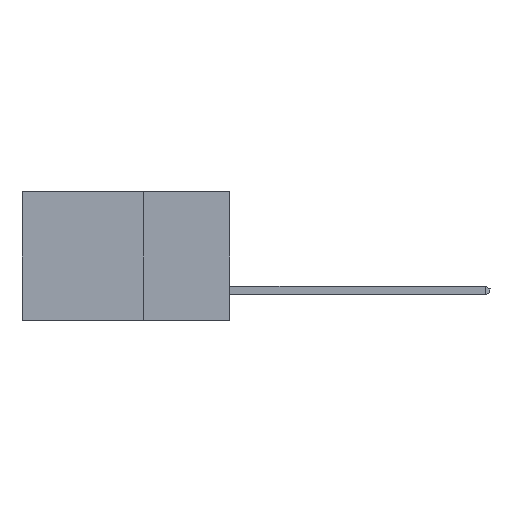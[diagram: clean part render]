
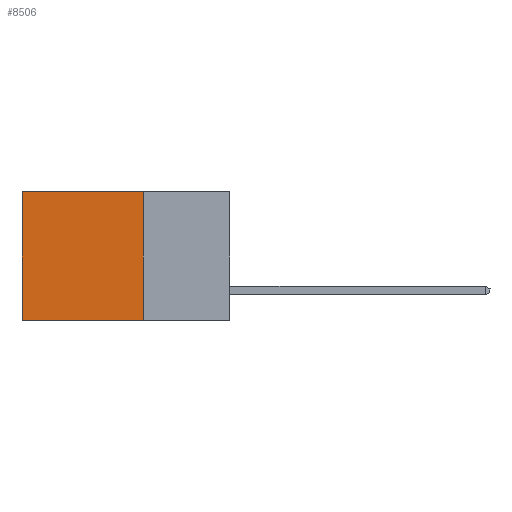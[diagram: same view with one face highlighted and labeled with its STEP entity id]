
A CAD part, left-side view. The second image highlights one B-rep face of the part: STEP entity #8506.
In plain terms, the highlighted planar face has unit normal (-1, 0, 0).
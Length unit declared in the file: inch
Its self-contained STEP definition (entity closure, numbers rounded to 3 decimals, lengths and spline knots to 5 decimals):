
#11 = EDGE_CURVE ( 'NONE', #2244, #3893, #8673, .T. ) ;
#474 = VECTOR ( 'NONE', #10063, 39.37008 ) ;
#539 = CARTESIAN_POINT ( 'NONE',  ( 0.2615, 0.25, -0.37 ) ) ;
#571 = LINE ( 'NONE', #3663, #9584 ) ;
#933 = LINE ( 'NONE', #4939, #4636 ) ;
#1692 = DIRECTION ( 'NONE',  ( 1., 0., 0. ) ) ;
#1859 = EDGE_CURVE ( 'NONE', #2244, #2149, #933, .T. ) ;
#2149 = VERTEX_POINT ( 'NONE', #4140 ) ;
#2244 = VERTEX_POINT ( 'NONE', #7410 ) ;
#2729 = ORIENTED_EDGE ( 'NONE', *, *, #6774, .T. ) ;
#2737 = CARTESIAN_POINT ( 'NONE',  ( 0.2615, 0.25, -0.37 ) ) ;
#2770 = DIRECTION ( 'NONE',  ( 0., 1., 0. ) ) ;
#2777 = CARTESIAN_POINT ( 'NONE',  ( 0.2615, 0.6, -0.37 ) ) ;
#3311 = EDGE_LOOP ( 'NONE', ( #2729, #11397, #3771, #11235 ) ) ;
#3663 = CARTESIAN_POINT ( 'NONE',  ( 0.2615, 0.6, -0.37 ) ) ;
#3712 = PLANE ( 'NONE',  #9403 ) ;
#3771 = ORIENTED_EDGE ( 'NONE', *, *, #11, .F. ) ;
#3893 = VERTEX_POINT ( 'NONE', #11339 ) ;
#4140 = CARTESIAN_POINT ( 'NONE',  ( 0.2615, 0.6, 0. ) ) ;
#4167 = EDGE_CURVE ( 'NONE', #3893, #5742, #5219, .T. ) ;
#4636 = VECTOR ( 'NONE', #2770, 39.37008 ) ;
#4939 = CARTESIAN_POINT ( 'NONE',  ( 0.2615, 0.25, 0. ) ) ;
#5219 = LINE ( 'NONE', #11192, #474 ) ;
#5742 = VERTEX_POINT ( 'NONE', #2777 ) ;
#6774 = EDGE_CURVE ( 'NONE', #2149, #5742, #571, .T. ) ;
#7410 = CARTESIAN_POINT ( 'NONE',  ( 0.2615, 0.25, 0. ) ) ;
#8486 = DIRECTION ( 'NONE',  ( 0., 0., -1. ) ) ;
#8506 = ADVANCED_FACE ( 'NONE', ( #12841 ), #3712, .F. ) ;
#8576 = DIRECTION ( 'NONE',  ( 0., 0., -1. ) ) ;
#8673 = LINE ( 'NONE', #539, #11702 ) ;
#9403 = AXIS2_PLACEMENT_3D ( 'NONE', #2737, #1692, #10802 ) ;
#9584 = VECTOR ( 'NONE', #8576, 39.37008 ) ;
#10063 = DIRECTION ( 'NONE',  ( 0., 1., 0. ) ) ;
#10802 = DIRECTION ( 'NONE',  ( 0., 0., -1. ) ) ;
#11192 = CARTESIAN_POINT ( 'NONE',  ( 0.2615, 0.25, -0.37 ) ) ;
#11235 = ORIENTED_EDGE ( 'NONE', *, *, #1859, .T. ) ;
#11339 = CARTESIAN_POINT ( 'NONE',  ( 0.2615, 0.25, -0.37 ) ) ;
#11397 = ORIENTED_EDGE ( 'NONE', *, *, #4167, .F. ) ;
#11702 = VECTOR ( 'NONE', #8486, 39.37008 ) ;
#12841 = FACE_OUTER_BOUND ( 'NONE', #3311, .T. ) ;
